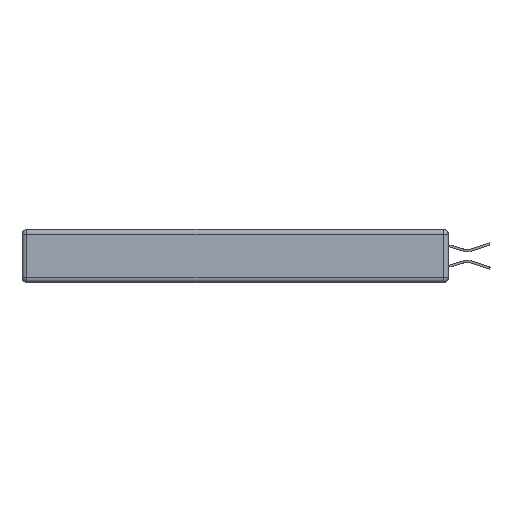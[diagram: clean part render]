
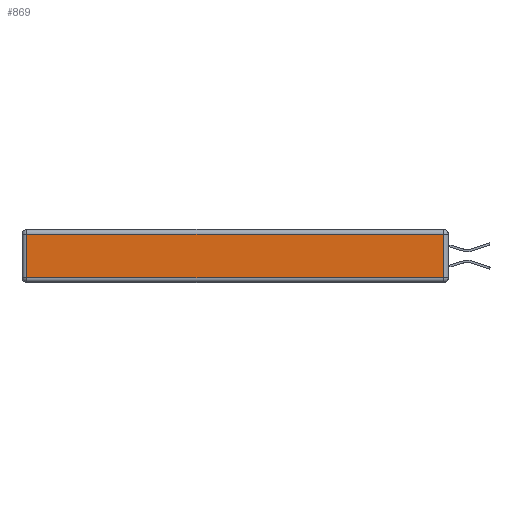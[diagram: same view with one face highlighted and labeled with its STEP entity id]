
A CAD part, left-side view. The second image highlights one B-rep face of the part: STEP entity #869.
In plain terms, the highlighted planar face has unit normal (-1, 0, 0).
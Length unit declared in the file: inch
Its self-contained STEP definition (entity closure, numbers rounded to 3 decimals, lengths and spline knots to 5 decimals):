
#228 = VECTOR ( 'NONE', #4947, 39.37008 ) ;
#869 = ADVANCED_FACE ( 'NONE', ( #2123 ), #13767, .T. ) ;
#2123 = FACE_OUTER_BOUND ( 'NONE', #11011, .T. ) ;
#2369 = VERTEX_POINT ( 'NONE', #9499 ) ;
#2477 = ORIENTED_EDGE ( 'NONE', *, *, #18655, .T. ) ;
#2822 = EDGE_CURVE ( 'NONE', #18962, #4099, #20585, .T. ) ;
#2977 = VECTOR ( 'NONE', #20140, 39.37008 ) ;
#3103 = LINE ( 'NONE', #19291, #11597 ) ;
#4099 = VERTEX_POINT ( 'NONE', #16785 ) ;
#4947 = DIRECTION ( 'NONE',  ( 0., 1., 0. ) ) ;
#4999 = DIRECTION ( 'NONE',  ( -1., 0., 0. ) ) ;
#7535 = LINE ( 'NONE', #16517, #2977 ) ;
#8224 = CARTESIAN_POINT ( 'NONE',  ( 0., 0.03, -0.343 ) ) ;
#8308 = AXIS2_PLACEMENT_3D ( 'NONE', #20528, #4999, #16838 ) ;
#9132 = VERTEX_POINT ( 'NONE', #15115 ) ;
#9393 = CARTESIAN_POINT ( 'NONE',  ( 0., 0.03, -0.313 ) ) ;
#9499 = CARTESIAN_POINT ( 'NONE',  ( 0., 2.72, -0.313 ) ) ;
#11011 = EDGE_LOOP ( 'NONE', ( #21828, #16203, #21015, #2477 ) ) ;
#11597 = VECTOR ( 'NONE', #19364, 39.37008 ) ;
#13767 = PLANE ( 'NONE',  #8308 ) ;
#15115 = CARTESIAN_POINT ( 'NONE',  ( 0., 2.72, -0.03 ) ) ;
#16203 = ORIENTED_EDGE ( 'NONE', *, *, #2822, .T. ) ;
#16517 = CARTESIAN_POINT ( 'NONE',  ( 0., 2.72, -0.343 ) ) ;
#16785 = CARTESIAN_POINT ( 'NONE',  ( 0., 0.03, -0.03 ) ) ;
#16838 = DIRECTION ( 'NONE',  ( 0., 0., 1. ) ) ;
#17680 = VECTOR ( 'NONE', #18821, 39.37008 ) ;
#18655 = EDGE_CURVE ( 'NONE', #9132, #2369, #7535, .T. ) ;
#18821 = DIRECTION ( 'NONE',  ( 0., 0., 1. ) ) ;
#18962 = VERTEX_POINT ( 'NONE', #9393 ) ;
#19291 = CARTESIAN_POINT ( 'NONE',  ( 0., 0., -0.313 ) ) ;
#19364 = DIRECTION ( 'NONE',  ( 0., -1., 0. ) ) ;
#19828 = LINE ( 'NONE', #20394, #228 ) ;
#20140 = DIRECTION ( 'NONE',  ( 0., 0., -1. ) ) ;
#20394 = CARTESIAN_POINT ( 'NONE',  ( 0., 2.75, -0.03 ) ) ;
#20471 = EDGE_CURVE ( 'NONE', #4099, #9132, #19828, .T. ) ;
#20528 = CARTESIAN_POINT ( 'NONE',  ( 0., 0., -0.343 ) ) ;
#20585 = LINE ( 'NONE', #8224, #17680 ) ;
#21015 = ORIENTED_EDGE ( 'NONE', *, *, #20471, .T. ) ;
#21097 = EDGE_CURVE ( 'NONE', #2369, #18962, #3103, .T. ) ;
#21828 = ORIENTED_EDGE ( 'NONE', *, *, #21097, .T. ) ;
